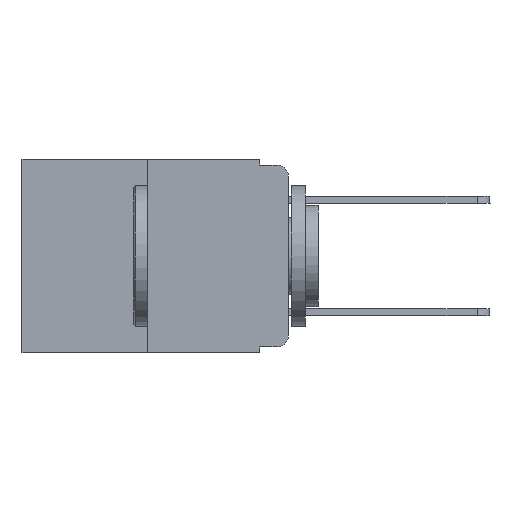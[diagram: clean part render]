
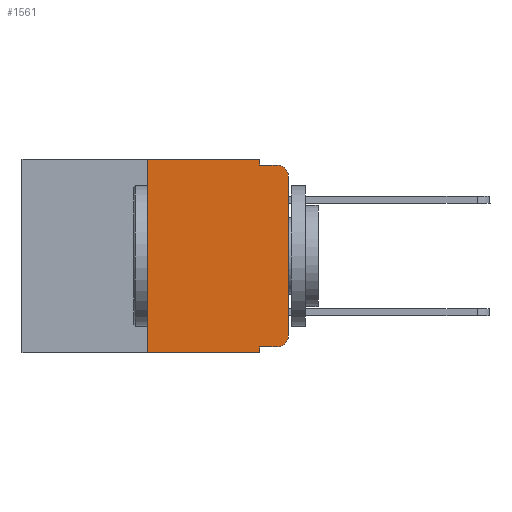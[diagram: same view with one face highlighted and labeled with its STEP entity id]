
A CAD part, left-side view. The second image highlights one B-rep face of the part: STEP entity #1561.
In plain terms, the highlighted planar face has unit normal (-1, 0, 0).
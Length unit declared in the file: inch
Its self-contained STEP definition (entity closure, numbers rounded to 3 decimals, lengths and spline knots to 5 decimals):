
#302 = EDGE_CURVE ( 'NONE', #1417, #7491, #2747, .T. ) ;
#466 = CARTESIAN_POINT ( 'NONE',  ( 0., 0.02, -0.03 ) ) ;
#502 = DIRECTION ( 'NONE',  ( -1., 0., 0. ) ) ;
#518 = DIRECTION ( 'NONE',  ( 0., -1., 0. ) ) ;
#572 = EDGE_CURVE ( 'NONE', #8997, #1148, #10029, .T. ) ;
#573 = CARTESIAN_POINT ( 'NONE',  ( 0., 0., -0.03 ) ) ;
#670 = VECTOR ( 'NONE', #6521, 39.37008 ) ;
#672 = LINE ( 'NONE', #2759, #670 ) ;
#1095 = CIRCLE ( 'NONE', #6118, 0.02 ) ;
#1148 = VERTEX_POINT ( 'NONE', #11084 ) ;
#1221 = VERTEX_POINT ( 'NONE', #11500 ) ;
#1233 = CARTESIAN_POINT ( 'NONE',  ( 0., 0.473, 0. ) ) ;
#1417 = VERTEX_POINT ( 'NONE', #2424 ) ;
#1467 = CARTESIAN_POINT ( 'NONE',  ( 0., 0.473, 0. ) ) ;
#1484 = DIRECTION ( 'NONE',  ( 0., 0., -1. ) ) ;
#1561 = ADVANCED_FACE ( 'NONE', ( #11683 ), #2198, .F. ) ;
#1655 = ORIENTED_EDGE ( 'NONE', *, *, #11469, .T. ) ;
#1707 = CARTESIAN_POINT ( 'NONE',  ( 0., 0.02, -0.313 ) ) ;
#1741 = CARTESIAN_POINT ( 'NONE',  ( 0., 0.051, -0.01 ) ) ;
#1844 = EDGE_CURVE ( 'NONE', #11035, #1221, #5209, .T. ) ;
#1934 = EDGE_CURVE ( 'NONE', #6318, #8997, #4354, .T. ) ;
#2045 = VECTOR ( 'NONE', #518, 39.37008 ) ;
#2198 = PLANE ( 'NONE',  #9764 ) ;
#2424 = CARTESIAN_POINT ( 'NONE',  ( 0., 0.051, -0.333 ) ) ;
#2528 = CARTESIAN_POINT ( 'NONE',  ( 0., 0.25, 0. ) ) ;
#2533 = DIRECTION ( 'NONE',  ( 0., 0., -1. ) ) ;
#2631 = ORIENTED_EDGE ( 'NONE', *, *, #10534, .T. ) ;
#2663 = CARTESIAN_POINT ( 'NONE',  ( 0., 0.051, -0.333 ) ) ;
#2673 = ORIENTED_EDGE ( 'NONE', *, *, #302, .F. ) ;
#2687 = DIRECTION ( 'NONE',  ( 1., 0., 0. ) ) ;
#2698 = EDGE_CURVE ( 'NONE', #6318, #7491, #10829, .T. ) ;
#2747 = LINE ( 'NONE', #5446, #11212 ) ;
#2759 = CARTESIAN_POINT ( 'NONE',  ( 0., 0.051, 0. ) ) ;
#3297 = CARTESIAN_POINT ( 'NONE',  ( 0., 0.473, -0.343 ) ) ;
#3694 = CIRCLE ( 'NONE', #12247, 0.02 ) ;
#3967 = CARTESIAN_POINT ( 'NONE',  ( 0., 0.25, 0. ) ) ;
#4201 = VECTOR ( 'NONE', #7178, 39.37008 ) ;
#4304 = LINE ( 'NONE', #8973, #4201 ) ;
#4323 = DIRECTION ( 'NONE',  ( 0., 0., -1. ) ) ;
#4354 = LINE ( 'NONE', #2528, #8800 ) ;
#4449 = ORIENTED_EDGE ( 'NONE', *, *, #2698, .T. ) ;
#4494 = LINE ( 'NONE', #2663, #6586 ) ;
#5046 = CARTESIAN_POINT ( 'NONE',  ( 0., 0.02, -0.333 ) ) ;
#5162 = VERTEX_POINT ( 'NONE', #5046 ) ;
#5209 = LINE ( 'NONE', #9015, #11771 ) ;
#5261 = VERTEX_POINT ( 'NONE', #573 ) ;
#5446 = CARTESIAN_POINT ( 'NONE',  ( 0., 0.051, 0. ) ) ;
#6118 = AXIS2_PLACEMENT_3D ( 'NONE', #1707, #502, #2533 ) ;
#6131 = CARTESIAN_POINT ( 'NONE',  ( 0., 0.25, -0.343 ) ) ;
#6318 = VERTEX_POINT ( 'NONE', #6131 ) ;
#6505 = EDGE_CURVE ( 'NONE', #1417, #5162, #4494, .T. ) ;
#6521 = DIRECTION ( 'NONE',  ( 0., 0., -1. ) ) ;
#6586 = VECTOR ( 'NONE', #7548, 39.37008 ) ;
#6620 = ORIENTED_EDGE ( 'NONE', *, *, #6505, .T. ) ;
#6911 = ORIENTED_EDGE ( 'NONE', *, *, #572, .F. ) ;
#6984 = ORIENTED_EDGE ( 'NONE', *, *, #1844, .F. ) ;
#7016 = EDGE_CURVE ( 'NONE', #10613, #5261, #4304, .T. ) ;
#7109 = DIRECTION ( 'NONE',  ( 0., -1., 0. ) ) ;
#7178 = DIRECTION ( 'NONE',  ( 0., 0., 1. ) ) ;
#7390 = EDGE_LOOP ( 'NONE', ( #11721, #1655, #6984, #9869, #6911, #11952, #4449, #2673, #6620, #2631 ) ) ;
#7491 = VERTEX_POINT ( 'NONE', #11877 ) ;
#7548 = DIRECTION ( 'NONE',  ( 0., -1., 0. ) ) ;
#8056 = DIRECTION ( 'NONE',  ( -1., 0., 0. ) ) ;
#8800 = VECTOR ( 'NONE', #9340, 39.37008 ) ;
#8973 = CARTESIAN_POINT ( 'NONE',  ( 0., 0., 0. ) ) ;
#8997 = VERTEX_POINT ( 'NONE', #3967 ) ;
#9015 = CARTESIAN_POINT ( 'NONE',  ( 0., 0.051, -0.01 ) ) ;
#9340 = DIRECTION ( 'NONE',  ( 0., 0., 1. ) ) ;
#9472 = VECTOR ( 'NONE', #7109, 39.37008 ) ;
#9764 = AXIS2_PLACEMENT_3D ( 'NONE', #1233, #2687, #1484 ) ;
#9869 = ORIENTED_EDGE ( 'NONE', *, *, #11147, .F. ) ;
#10029 = LINE ( 'NONE', #1467, #2045 ) ;
#10308 = DIRECTION ( 'NONE',  ( 0., 0., -1. ) ) ;
#10534 = EDGE_CURVE ( 'NONE', #5162, #10613, #1095, .T. ) ;
#10613 = VERTEX_POINT ( 'NONE', #11946 ) ;
#10829 = LINE ( 'NONE', #3297, #9472 ) ;
#11035 = VERTEX_POINT ( 'NONE', #1741 ) ;
#11084 = CARTESIAN_POINT ( 'NONE',  ( 0., 0.051, 0. ) ) ;
#11147 = EDGE_CURVE ( 'NONE', #1148, #11035, #672, .T. ) ;
#11212 = VECTOR ( 'NONE', #10308, 39.37008 ) ;
#11469 = EDGE_CURVE ( 'NONE', #5261, #1221, #3694, .T. ) ;
#11500 = CARTESIAN_POINT ( 'NONE',  ( 0., 0.02, -0.01 ) ) ;
#11683 = FACE_OUTER_BOUND ( 'NONE', #7390, .T. ) ;
#11721 = ORIENTED_EDGE ( 'NONE', *, *, #7016, .T. ) ;
#11763 = DIRECTION ( 'NONE',  ( 0., -1., 0. ) ) ;
#11771 = VECTOR ( 'NONE', #11763, 39.37008 ) ;
#11877 = CARTESIAN_POINT ( 'NONE',  ( 0., 0.051, -0.343 ) ) ;
#11946 = CARTESIAN_POINT ( 'NONE',  ( 0., 0., -0.313 ) ) ;
#11952 = ORIENTED_EDGE ( 'NONE', *, *, #1934, .F. ) ;
#12247 = AXIS2_PLACEMENT_3D ( 'NONE', #466, #8056, #4323 ) ;
